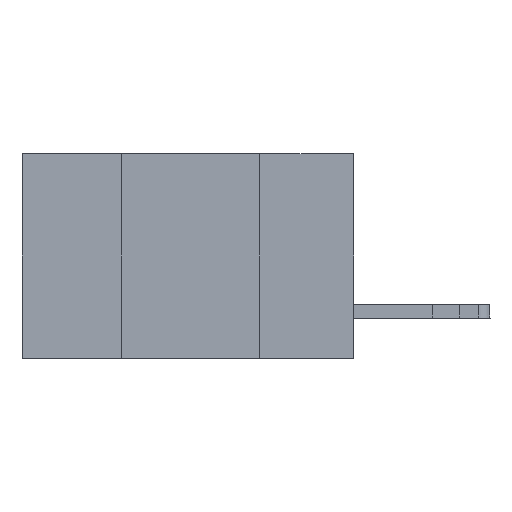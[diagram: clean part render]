
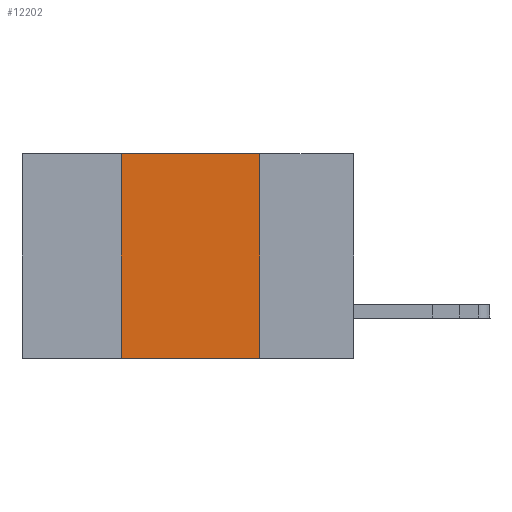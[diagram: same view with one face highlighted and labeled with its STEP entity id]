
A CAD part, left-side view. The second image highlights one B-rep face of the part: STEP entity #12202.
In plain terms, the highlighted planar face has unit normal (-1, 0, 0).
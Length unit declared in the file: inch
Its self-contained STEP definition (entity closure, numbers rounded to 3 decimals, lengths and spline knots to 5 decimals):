
#1220 = EDGE_CURVE ( 'NONE', #2351, #12336, #11265, .T. ) ;
#2351 = VERTEX_POINT ( 'NONE', #9408 ) ;
#2360 = CARTESIAN_POINT ( 'NONE',  ( 0., 0.17, 0. ) ) ;
#2928 = CARTESIAN_POINT ( 'NONE',  ( 0., 0.42, 0. ) ) ;
#3346 = EDGE_CURVE ( 'NONE', #12336, #8203, #16885, .T. ) ;
#3556 = ORIENTED_EDGE ( 'NONE', *, *, #8972, .T. ) ;
#3952 = CARTESIAN_POINT ( 'NONE',  ( 0., 0.17, 0. ) ) ;
#4584 = EDGE_CURVE ( 'NONE', #8203, #5917, #10375, .T. ) ;
#5917 = VERTEX_POINT ( 'NONE', #11537 ) ;
#8203 = VERTEX_POINT ( 'NONE', #3952 ) ;
#8652 = CARTESIAN_POINT ( 'NONE',  ( 0., 0.6, 0. ) ) ;
#8718 = LINE ( 'NONE', #9248, #14160 ) ;
#8972 = EDGE_CURVE ( 'NONE', #2351, #5917, #8718, .T. ) ;
#9248 = CARTESIAN_POINT ( 'NONE',  ( 0., 0.6, -0.37 ) ) ;
#9408 = CARTESIAN_POINT ( 'NONE',  ( 0., 0.42, -0.37 ) ) ;
#10020 = DIRECTION ( 'NONE',  ( 0., -1., 0. ) ) ;
#10085 = ORIENTED_EDGE ( 'NONE', *, *, #1220, .F. ) ;
#10375 = LINE ( 'NONE', #2360, #12560 ) ;
#10979 = CARTESIAN_POINT ( 'NONE',  ( 0., 0.6, 0. ) ) ;
#11265 = LINE ( 'NONE', #2928, #13217 ) ;
#11319 = DIRECTION ( 'NONE',  ( 0., 0., 1. ) ) ;
#11537 = CARTESIAN_POINT ( 'NONE',  ( 0., 0.17, -0.37 ) ) ;
#11684 = CARTESIAN_POINT ( 'NONE',  ( 0., 0.42, 0. ) ) ;
#12202 = ADVANCED_FACE ( 'NONE', ( #14592 ), #12241, .F. ) ;
#12241 = PLANE ( 'NONE',  #14393 ) ;
#12336 = VERTEX_POINT ( 'NONE', #11684 ) ;
#12560 = VECTOR ( 'NONE', #13434, 39.37008 ) ;
#12997 = EDGE_LOOP ( 'NONE', ( #16158, #17259, #10085, #3556 ) ) ;
#13217 = VECTOR ( 'NONE', #11319, 39.37008 ) ;
#13434 = DIRECTION ( 'NONE',  ( 0., 0., -1. ) ) ;
#13701 = DIRECTION ( 'NONE',  ( 1., 0., 0. ) ) ;
#14160 = VECTOR ( 'NONE', #16215, 39.37008 ) ;
#14393 = AXIS2_PLACEMENT_3D ( 'NONE', #10979, #13701, #16537 ) ;
#14592 = FACE_OUTER_BOUND ( 'NONE', #12997, .T. ) ;
#16158 = ORIENTED_EDGE ( 'NONE', *, *, #4584, .F. ) ;
#16215 = DIRECTION ( 'NONE',  ( 0., -1., 0. ) ) ;
#16451 = VECTOR ( 'NONE', #10020, 39.37008 ) ;
#16537 = DIRECTION ( 'NONE',  ( 0., 0., -1. ) ) ;
#16885 = LINE ( 'NONE', #8652, #16451 ) ;
#17259 = ORIENTED_EDGE ( 'NONE', *, *, #3346, .F. ) ;
